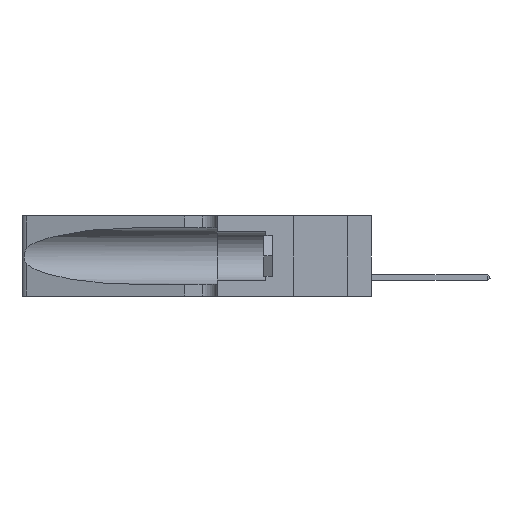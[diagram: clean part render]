
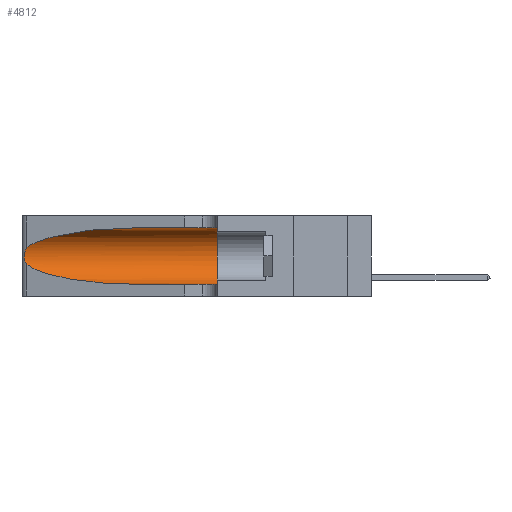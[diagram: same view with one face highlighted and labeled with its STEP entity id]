
A CAD part, left-side view. The second image highlights one B-rep face of the part: STEP entity #4812.
In plain terms, the highlighted cylindrical face has radius 3.308 mm (diameter 6.617 mm), a partial arc.
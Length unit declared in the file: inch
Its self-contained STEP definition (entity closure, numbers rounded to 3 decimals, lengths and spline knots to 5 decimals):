
#112 = ORIENTED_EDGE ( 'NONE', *, *, #34001, .T. ) ;
#1840 = CARTESIAN_POINT ( 'NONE',  ( 0.1305, 1.61858, 0.05475 ) ) ;
#2575 = CARTESIAN_POINT ( 'NONE',  ( 0.1305, 0.35, 0.185 ) ) ;
#2755 = B_SPLINE_CURVE_WITH_KNOTS ( 'NONE', 3,
 ( #28900, #36383, #6447, #13537, #9892, #17713, #39882, #36554, #21403, #44437, #13194, #13722, #43896, #36211 ),
 .UNSPECIFIED., .F., .F.,
 ( 4, 2, 2, 2, 2, 2, 4 ),
 ( 0., 0.00027, 0.00053, 0.00107, 0.0016, 0.00187, 0.00214 ),
 .UNSPECIFIED. ) ;
#4305 = VECTOR ( 'NONE', #44086, 39.37008 ) ;
#4793 = ORIENTED_EDGE ( 'NONE', *, *, #36015, .T. ) ;
#4812 = ADVANCED_FACE ( 'NONE', ( #38445 ), #26602, .F. ) ;
#5133 = CARTESIAN_POINT ( 'NONE',  ( 0.2373, 1.15595, 0.28018 ) ) ;
#6447 = CARTESIAN_POINT ( 'NONE',  ( 0.25639, 1.23184, 0.21858 ) ) ;
#6577 = ORIENTED_EDGE ( 'NONE', *, *, #42695, .T. ) ;
#6587 = DIRECTION ( 'NONE',  ( 0., 0., 1. ) ) ;
#8152 = VERTEX_POINT ( 'NONE', #14553 ) ;
#8709 = AXIS2_PLACEMENT_3D ( 'NONE', #43790, #27792, #24114 ) ;
#8855 = CARTESIAN_POINT ( 'NONE',  ( 0.1305, 0.72297, 0.31525 ) ) ;
#9406 = CARTESIAN_POINT ( 'NONE',  ( 0.1305, 0.72297, 0.31525 ) ) ;
#9892 = CARTESIAN_POINT ( 'NONE',  ( 0.25854, 1.2359, 0.20912 ) ) ;
#10060 = VERTEX_POINT ( 'NONE', #46717 ) ;
#10366 = CARTESIAN_POINT ( 'NONE',  ( 0.18966, 0.96281, 0.05475 ) ) ;
#10719 = DIRECTION ( 'NONE',  ( 0., 1., 0. ) ) ;
#11555 =( BOUNDED_CURVE ( )  B_SPLINE_CURVE ( 3, ( #8855, #39092, #5133, #31764 ),
 .UNSPECIFIED., .F., .T. ) 
 B_SPLINE_CURVE_WITH_KNOTS ( ( 4, 4 ),
 ( 1.5708, 2.84003 ),
 .UNSPECIFIED. ) 
 CURVE ( )  GEOMETRIC_REPRESENTATION_ITEM ( )  RATIONAL_B_SPLINE_CURVE ( ( 1., 0.87, 0.87, 1. ) ) 
 REPRESENTATION_ITEM ( '' )  );
#13194 = CARTESIAN_POINT ( 'NONE',  ( 0.25789, 1.23486, 0.15765 ) ) ;
#13537 = CARTESIAN_POINT ( 'NONE',  ( 0.25787, 1.23484, 0.2124 ) ) ;
#13722 = CARTESIAN_POINT ( 'NONE',  ( 0.25639, 1.23186, 0.15144 ) ) ;
#14389 = EDGE_CURVE ( 'NONE', #17086, #8152, #45477, .T. ) ;
#14553 = CARTESIAN_POINT ( 'NONE',  ( 0.1305, 0.35, 0.31525 ) ) ;
#15136 = VERTEX_POINT ( 'NONE', #33620 ) ;
#16946 = EDGE_LOOP ( 'NONE', ( #37473, #6577, #112, #4793, #23794, #29810 ) ) ;
#17086 = VERTEX_POINT ( 'NONE', #9406 ) ;
#17713 = CARTESIAN_POINT ( 'NONE',  ( 0.26018, 1.23835, 0.19895 ) ) ;
#18381 = CARTESIAN_POINT ( 'NONE',  ( 0.25487, 1.22718, 0.14631 ) ) ;
#21257 = LINE ( 'NONE', #1840, #29015 ) ;
#21403 = CARTESIAN_POINT ( 'NONE',  ( 0.26017, 1.23833, 0.17102 ) ) ;
#23209 = CARTESIAN_POINT ( 'NONE',  ( 0.25487, 1.22718, 0.14631 ) ) ;
#23794 = ORIENTED_EDGE ( 'NONE', *, *, #36267, .F. ) ;
#24114 = DIRECTION ( 'NONE',  ( 0., 0., -1. ) ) ;
#25028 = DIRECTION ( 'NONE',  ( 0., -1., 0. ) ) ;
#26602 = CYLINDRICAL_SURFACE ( 'NONE', #8709, 0.13025 ) ;
#27199 = CIRCLE ( 'NONE', #49089, 0.13025 ) ;
#27792 = DIRECTION ( 'NONE',  ( 0., -1., 0. ) ) ;
#28900 = CARTESIAN_POINT ( 'NONE',  ( 0.25487, 1.22718, 0.22369 ) ) ;
#29015 = VECTOR ( 'NONE', #25028, 39.37008 ) ;
#29312 =( BOUNDED_CURVE ( )  B_SPLINE_CURVE ( 3, ( #18381, #40535, #10366, #40715 ),
 .UNSPECIFIED., .F., .F. ) 
 B_SPLINE_CURVE_WITH_KNOTS ( ( 4, 4 ),
 ( 3.44316, 4.71239 ),
 .UNSPECIFIED. ) 
 CURVE ( )  GEOMETRIC_REPRESENTATION_ITEM ( )  RATIONAL_B_SPLINE_CURVE ( ( 1., 0.87, 0.87, 1. ) ) 
 REPRESENTATION_ITEM ( '' )  );
#29810 = ORIENTED_EDGE ( 'NONE', *, *, #14389, .F. ) ;
#31764 = CARTESIAN_POINT ( 'NONE',  ( 0.25487, 1.22718, 0.22369 ) ) ;
#33620 = CARTESIAN_POINT ( 'NONE',  ( 0.25487, 1.22718, 0.22369 ) ) ;
#34001 = EDGE_CURVE ( 'NONE', #40368, #10060, #29312, .T. ) ;
#36015 = EDGE_CURVE ( 'NONE', #10060, #41160, #21257, .T. ) ;
#36211 = CARTESIAN_POINT ( 'NONE',  ( 0.25487, 1.22718, 0.14631 ) ) ;
#36267 = EDGE_CURVE ( 'NONE', #8152, #41160, #27199, .T. ) ;
#36383 = CARTESIAN_POINT ( 'NONE',  ( 0.25555, 1.22994, 0.2215 ) ) ;
#36400 = CARTESIAN_POINT ( 'NONE',  ( 0.1305, 1.61858, 0.31525 ) ) ;
#36554 = CARTESIAN_POINT ( 'NONE',  ( 0.26075, 1.23896, 0.178 ) ) ;
#37473 = ORIENTED_EDGE ( 'NONE', *, *, #40287, .T. ) ;
#38113 = CARTESIAN_POINT ( 'NONE',  ( 0.1305, 0.35, 0.05475 ) ) ;
#38445 = FACE_OUTER_BOUND ( 'NONE', #16946, .T. ) ;
#39092 = CARTESIAN_POINT ( 'NONE',  ( 0.18966, 0.96281, 0.31525 ) ) ;
#39882 = CARTESIAN_POINT ( 'NONE',  ( 0.26075, 1.23896, 0.19203 ) ) ;
#40287 = EDGE_CURVE ( 'NONE', #17086, #15136, #11555, .T. ) ;
#40368 = VERTEX_POINT ( 'NONE', #23209 ) ;
#40535 = CARTESIAN_POINT ( 'NONE',  ( 0.2373, 1.15595, 0.08982 ) ) ;
#40715 = CARTESIAN_POINT ( 'NONE',  ( 0.1305, 0.72297, 0.05475 ) ) ;
#41160 = VERTEX_POINT ( 'NONE', #38113 ) ;
#42695 = EDGE_CURVE ( 'NONE', #15136, #40368, #2755, .T. ) ;
#43790 = CARTESIAN_POINT ( 'NONE',  ( 0.1305, 1.61858, 0.185 ) ) ;
#43896 = CARTESIAN_POINT ( 'NONE',  ( 0.25555, 1.22993, 0.14849 ) ) ;
#44086 = DIRECTION ( 'NONE',  ( 0., -1., 0. ) ) ;
#44437 = CARTESIAN_POINT ( 'NONE',  ( 0.25856, 1.23593, 0.16098 ) ) ;
#45477 = LINE ( 'NONE', #36400, #4305 ) ;
#46717 = CARTESIAN_POINT ( 'NONE',  ( 0.1305, 0.72297, 0.05475 ) ) ;
#49089 = AXIS2_PLACEMENT_3D ( 'NONE', #2575, #10719, #6587 ) ;
